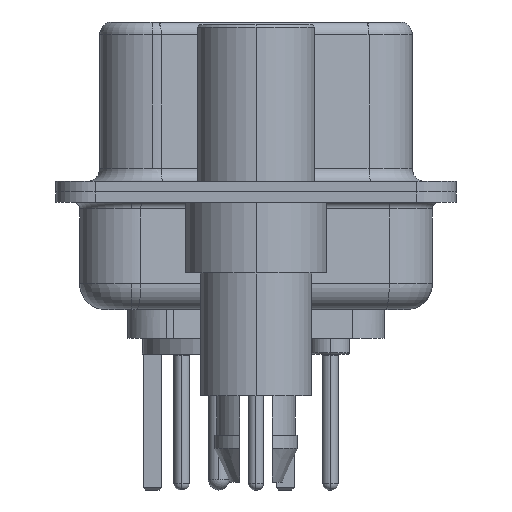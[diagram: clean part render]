
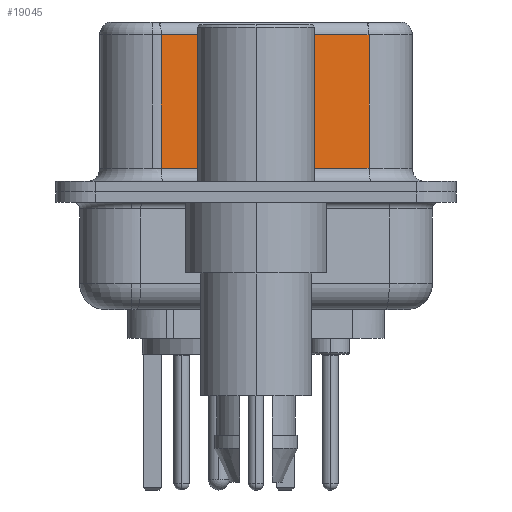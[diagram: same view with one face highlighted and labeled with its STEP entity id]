
A CAD part, left-side view. The second image highlights one B-rep face of the part: STEP entity #19045.
In plain terms, the highlighted planar face has unit normal (-0.985, -0.174, 0).
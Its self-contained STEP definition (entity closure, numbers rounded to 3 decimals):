
#78 = EDGE_CURVE ( 'NONE', #25757, #28083, #27994, .T. ) ;
#521 = CARTESIAN_POINT ( 'NONE',  ( 3.73, 3.628, 0.9 ) ) ;
#962 = CARTESIAN_POINT ( 'NONE',  ( 3.73, 3.628, 6.52 ) ) ;
#1104 = FACE_OUTER_BOUND ( 'NONE', #25024, .T. ) ;
#2188 = AXIS2_PLACEMENT_3D ( 'NONE', #30915, #26017, #11012 ) ;
#2994 = VECTOR ( 'NONE', #12790, 1000. ) ;
#4095 = CARTESIAN_POINT ( 'NONE',  ( 5.132, -4.322, 6.02 ) ) ;
#4141 = EDGE_CURVE ( 'NONE', #20166, #22434, #23000, .T. ) ;
#5244 = CARTESIAN_POINT ( 'NONE',  ( 5.132, -4.322, 0.9 ) ) ;
#5948 = PLANE ( 'NONE',  #2188 ) ;
#6794 = ORIENTED_EDGE ( 'NONE', *, *, #4141, .T. ) ;
#7758 = DIRECTION ( 'NONE',  ( 0., 0., -1. ) ) ;
#8023 = VECTOR ( 'NONE', #30114, 1000. ) ;
#11012 = DIRECTION ( 'NONE',  ( -0.174, 0.985, 0. ) ) ;
#12716 = CARTESIAN_POINT ( 'NONE',  ( 3.73, 3.628, 6.02 ) ) ;
#12790 = DIRECTION ( 'NONE',  ( 0.174, -0.985, 0. ) ) ;
#14373 = ORIENTED_EDGE ( 'NONE', *, *, #16771, .T. ) ;
#15196 = CARTESIAN_POINT ( 'NONE',  ( 5.132, -4.322, 6.52 ) ) ;
#15673 = LINE ( 'NONE', #962, #28216 ) ;
#16051 = LINE ( 'NONE', #15196, #22744 ) ;
#16771 = EDGE_CURVE ( 'NONE', #28083, #20166, #15673, .T. ) ;
#18501 = DIRECTION ( 'NONE',  ( 0., 0., -1. ) ) ;
#19045 = ADVANCED_FACE ( 'NONE', ( #1104 ), #5948, .F. ) ;
#20023 = CARTESIAN_POINT ( 'NONE',  ( 5.132, -4.322, 0.9 ) ) ;
#20166 = VERTEX_POINT ( 'NONE', #521 ) ;
#22257 = CARTESIAN_POINT ( 'NONE',  ( 5.132, -4.322, 6.02 ) ) ;
#22434 = VERTEX_POINT ( 'NONE', #20023 ) ;
#22744 = VECTOR ( 'NONE', #7758, 1000. ) ;
#22960 = ORIENTED_EDGE ( 'NONE', *, *, #78, .T. ) ;
#23000 = LINE ( 'NONE', #5244, #2994 ) ;
#25024 = EDGE_LOOP ( 'NONE', ( #28641, #22960, #14373, #6794 ) ) ;
#25757 = VERTEX_POINT ( 'NONE', #22257 ) ;
#26017 = DIRECTION ( 'NONE',  ( 0.985, 0.174, 0. ) ) ;
#27994 = LINE ( 'NONE', #4095, #8023 ) ;
#28083 = VERTEX_POINT ( 'NONE', #12716 ) ;
#28216 = VECTOR ( 'NONE', #18501, 1000. ) ;
#28641 = ORIENTED_EDGE ( 'NONE', *, *, #29226, .F. ) ;
#29226 = EDGE_CURVE ( 'NONE', #25757, #22434, #16051, .T. ) ;
#30114 = DIRECTION ( 'NONE',  ( -0.174, 0.985, 0. ) ) ;
#30915 = CARTESIAN_POINT ( 'NONE',  ( 5.132, -4.322, 6.52 ) ) ;
